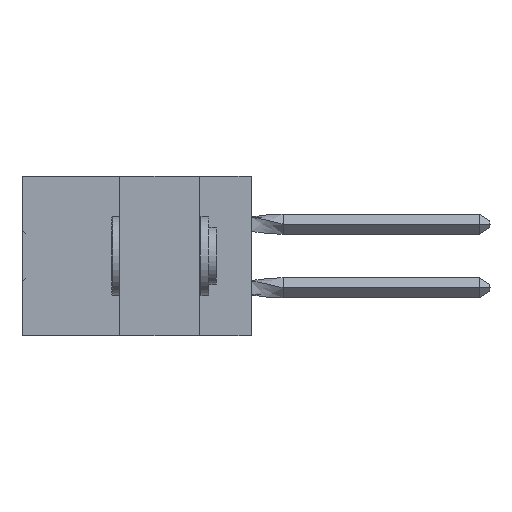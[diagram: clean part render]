
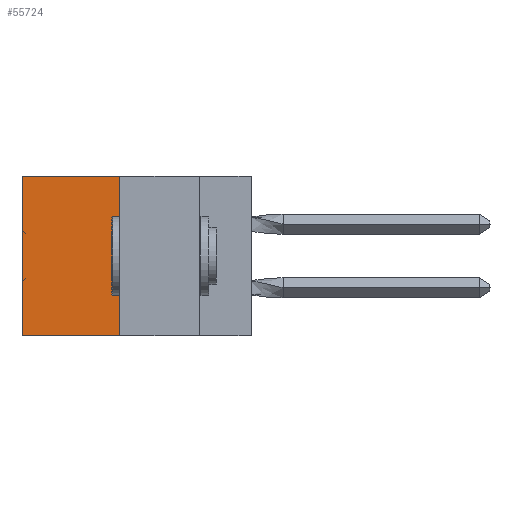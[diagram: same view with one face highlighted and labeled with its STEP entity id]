
A CAD part, left-side view. The second image highlights one B-rep face of the part: STEP entity #55724.
In plain terms, the highlighted planar face has unit normal (-1, 0, 0).
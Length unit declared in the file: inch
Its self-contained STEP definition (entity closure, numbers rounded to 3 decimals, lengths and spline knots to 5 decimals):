
#3172 = DIRECTION ( 'NONE',  ( 0., 0., -1. ) ) ;
#6300 = CARTESIAN_POINT ( 'NONE',  ( 0.305, 0.72, -0.5 ) ) ;
#7774 = VECTOR ( 'NONE', #15837, 39.37008 ) ;
#8648 = PLANE ( 'NONE',  #32781 ) ;
#9573 = ORIENTED_EDGE ( 'NONE', *, *, #19679, .F. ) ;
#9992 = CARTESIAN_POINT ( 'NONE',  ( 0.305, 0.413, 0. ) ) ;
#12384 = CARTESIAN_POINT ( 'NONE',  ( 0.305, 0.413, -0.5 ) ) ;
#12846 = LINE ( 'NONE', #6300, #7774 ) ;
#12970 = EDGE_CURVE ( 'NONE', #39527, #54892, #44445, .T. ) ;
#13490 = DIRECTION ( 'NONE',  ( 1., 0., 0. ) ) ;
#13690 = CARTESIAN_POINT ( 'NONE',  ( 0.305, 0.413, -0.5 ) ) ;
#14680 = DIRECTION ( 'NONE',  ( 0., 1., 0. ) ) ;
#15837 = DIRECTION ( 'NONE',  ( 0., 0., -1. ) ) ;
#16701 = EDGE_CURVE ( 'NONE', #39527, #40867, #24920, .T. ) ;
#19679 = EDGE_CURVE ( 'NONE', #54892, #38426, #27555, .T. ) ;
#20392 = DIRECTION ( 'NONE',  ( 0., 1., 0. ) ) ;
#20522 = EDGE_CURVE ( 'NONE', #40867, #38426, #12846, .T. ) ;
#20622 = ORIENTED_EDGE ( 'NONE', *, *, #12970, .F. ) ;
#20983 = ORIENTED_EDGE ( 'NONE', *, *, #16701, .T. ) ;
#24920 = LINE ( 'NONE', #44061, #26369 ) ;
#26369 = VECTOR ( 'NONE', #20392, 39.37008 ) ;
#27555 = LINE ( 'NONE', #46913, #37705 ) ;
#32014 = DIRECTION ( 'NONE',  ( 0., 0., -1. ) ) ;
#32781 = AXIS2_PLACEMENT_3D ( 'NONE', #13690, #13490, #32014 ) ;
#33536 = CARTESIAN_POINT ( 'NONE',  ( 0.305, 0.72, -0.5 ) ) ;
#37651 = CARTESIAN_POINT ( 'NONE',  ( 0.305, 0.72, 0. ) ) ;
#37705 = VECTOR ( 'NONE', #14680, 39.37008 ) ;
#38426 = VERTEX_POINT ( 'NONE', #33536 ) ;
#39527 = VERTEX_POINT ( 'NONE', #9992 ) ;
#40867 = VERTEX_POINT ( 'NONE', #37651 ) ;
#42464 = CARTESIAN_POINT ( 'NONE',  ( 0.305, 0.413, -0.5 ) ) ;
#42936 = FACE_OUTER_BOUND ( 'NONE', #46731, .T. ) ;
#44061 = CARTESIAN_POINT ( 'NONE',  ( 0.305, 0.413, 0. ) ) ;
#44445 = LINE ( 'NONE', #12384, #50262 ) ;
#46731 = EDGE_LOOP ( 'NONE', ( #48568, #9573, #20622, #20983 ) ) ;
#46913 = CARTESIAN_POINT ( 'NONE',  ( 0.305, 0.413, -0.5 ) ) ;
#48568 = ORIENTED_EDGE ( 'NONE', *, *, #20522, .T. ) ;
#50262 = VECTOR ( 'NONE', #3172, 39.37008 ) ;
#54892 = VERTEX_POINT ( 'NONE', #42464 ) ;
#55724 = ADVANCED_FACE ( 'NONE', ( #42936 ), #8648, .F. ) ;
